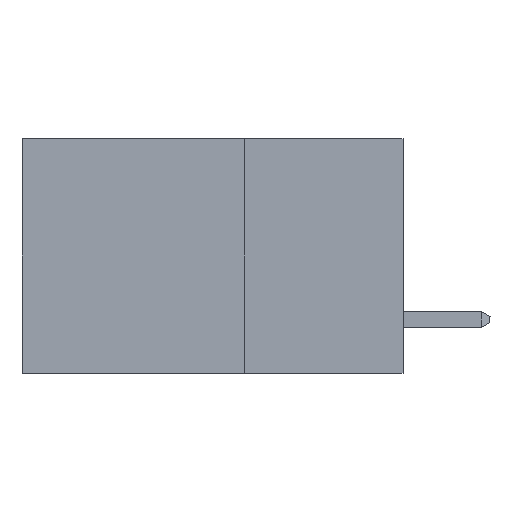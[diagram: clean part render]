
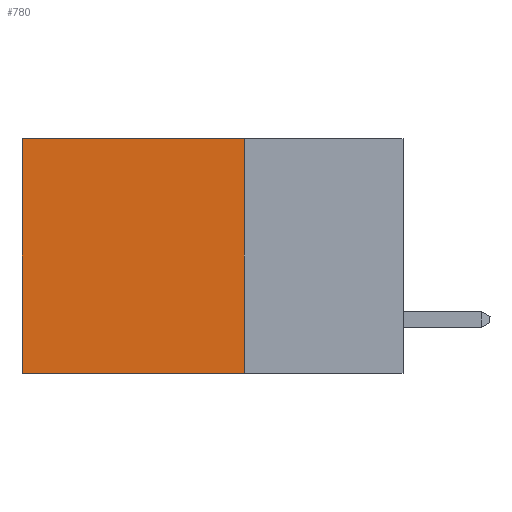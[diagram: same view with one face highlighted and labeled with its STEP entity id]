
A CAD part, left-side view. The second image highlights one B-rep face of the part: STEP entity #780.
In plain terms, the highlighted planar face has unit normal (-1, 0, 0).
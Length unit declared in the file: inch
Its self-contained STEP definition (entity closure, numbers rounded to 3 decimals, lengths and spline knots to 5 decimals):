
#780 = ADVANCED_FACE ( 'NONE', ( #30822 ), #31194, .F. ) ;
#2367 = ORIENTED_EDGE ( 'NONE', *, *, #36925, .F. ) ;
#2572 = CARTESIAN_POINT ( 'NONE',  ( 0.2875, 0.25, 0. ) ) ;
#2844 = ORIENTED_EDGE ( 'NONE', *, *, #25201, .T. ) ;
#2919 = LINE ( 'NONE', #31360, #6251 ) ;
#5441 = LINE ( 'NONE', #15093, #14253 ) ;
#5634 = ORIENTED_EDGE ( 'NONE', *, *, #27645, .F. ) ;
#6251 = VECTOR ( 'NONE', #23487, 39.37008 ) ;
#7072 = CARTESIAN_POINT ( 'NONE',  ( 0.2875, 0.6, -0.37 ) ) ;
#7891 = EDGE_CURVE ( 'NONE', #21448, #9490, #9098, .T. ) ;
#8824 = VECTOR ( 'NONE', #26850, 39.37008 ) ;
#8997 = CARTESIAN_POINT ( 'NONE',  ( 0.2875, 0.6, 0. ) ) ;
#9098 = LINE ( 'NONE', #31928, #8824 ) ;
#9490 = VERTEX_POINT ( 'NONE', #8997 ) ;
#10102 = VERTEX_POINT ( 'NONE', #7072 ) ;
#12457 = CARTESIAN_POINT ( 'NONE',  ( 0.2875, 0.6, 0. ) ) ;
#13523 = VECTOR ( 'NONE', #29676, 39.37008 ) ;
#14253 = VECTOR ( 'NONE', #28273, 39.37008 ) ;
#14340 = DIRECTION ( 'NONE',  ( 0., 0., -1. ) ) ;
#15093 = CARTESIAN_POINT ( 'NONE',  ( 0.2875, 0.25, -0.37 ) ) ;
#18136 = EDGE_LOOP ( 'NONE', ( #2844, #5634, #2367, #34938 ) ) ;
#19945 = DIRECTION ( 'NONE',  ( 1., 0., 0. ) ) ;
#20745 = AXIS2_PLACEMENT_3D ( 'NONE', #2572, #19945, #14340 ) ;
#21448 = VERTEX_POINT ( 'NONE', #31199 ) ;
#23487 = DIRECTION ( 'NONE',  ( 0., 0., -1. ) ) ;
#23878 = LINE ( 'NONE', #12457, #13523 ) ;
#25201 = EDGE_CURVE ( 'NONE', #9490, #10102, #23878, .T. ) ;
#26850 = DIRECTION ( 'NONE',  ( 0., 1., 0. ) ) ;
#27645 = EDGE_CURVE ( 'NONE', #35636, #10102, #5441, .T. ) ;
#28273 = DIRECTION ( 'NONE',  ( 0., 1., 0. ) ) ;
#29676 = DIRECTION ( 'NONE',  ( 0., 0., -1. ) ) ;
#30822 = FACE_OUTER_BOUND ( 'NONE', #18136, .T. ) ;
#31194 = PLANE ( 'NONE',  #20745 ) ;
#31199 = CARTESIAN_POINT ( 'NONE',  ( 0.2875, 0.25, 0. ) ) ;
#31360 = CARTESIAN_POINT ( 'NONE',  ( 0.2875, 0.25, 0. ) ) ;
#31928 = CARTESIAN_POINT ( 'NONE',  ( 0.2875, 0.25, 0. ) ) ;
#34938 = ORIENTED_EDGE ( 'NONE', *, *, #7891, .T. ) ;
#35636 = VERTEX_POINT ( 'NONE', #35737 ) ;
#35737 = CARTESIAN_POINT ( 'NONE',  ( 0.2875, 0.25, -0.37 ) ) ;
#36925 = EDGE_CURVE ( 'NONE', #21448, #35636, #2919, .T. ) ;
